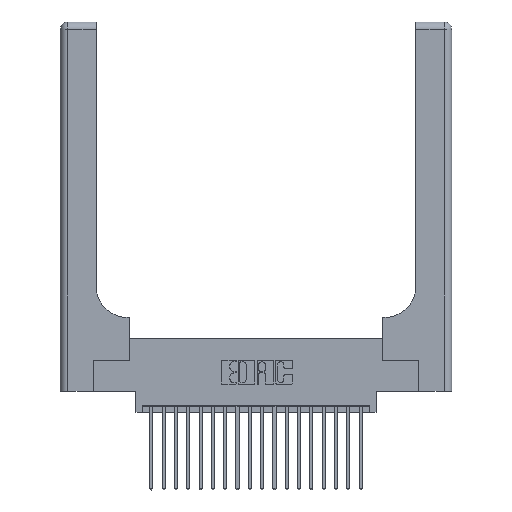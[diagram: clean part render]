
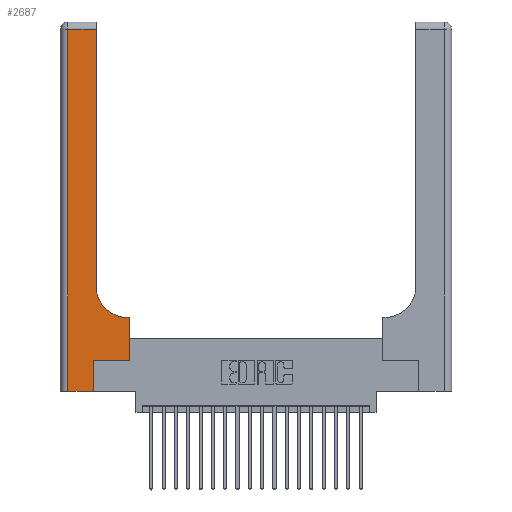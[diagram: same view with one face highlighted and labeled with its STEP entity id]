
A CAD part, top view. The second image highlights one B-rep face of the part: STEP entity #2687.
In plain terms, the highlighted planar face has unit normal (0, 0, 1).
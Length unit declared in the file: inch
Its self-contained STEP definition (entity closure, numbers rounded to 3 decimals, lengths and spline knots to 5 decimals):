
#293 = VECTOR ( 'NONE', #5653, 39.37008 ) ;
#334 = VECTOR ( 'NONE', #6214, 39.37008 ) ;
#410 = EDGE_CURVE ( 'NONE', #9413, #22531, #4582, .T. ) ;
#732 = AXIS2_PLACEMENT_3D ( 'NONE', #22303, #11913, #1393 ) ;
#791 = DIRECTION ( 'NONE',  ( 0., 0., -1. ) ) ;
#1054 = AXIS2_PLACEMENT_3D ( 'NONE', #16647, #791, #11550 ) ;
#1213 = CARTESIAN_POINT ( 'NONE',  ( 0.269, 0.25, 0.37 ) ) ;
#1229 = ORIENTED_EDGE ( 'NONE', *, *, #21513, .T. ) ;
#1301 = CARTESIAN_POINT ( 'NONE',  ( 0., 0., 0.37 ) ) ;
#1393 = DIRECTION ( 'NONE',  ( 1., 0., 0. ) ) ;
#1927 = CARTESIAN_POINT ( 'NONE',  ( 0.06, 3., 0.37 ) ) ;
#2687 = ADVANCED_FACE ( 'NONE', ( #8909 ), #16555, .F. ) ;
#2688 = CIRCLE ( 'NONE', #732, 0.25 ) ;
#2940 = VECTOR ( 'NONE', #15321, 39.37008 ) ;
#3001 = EDGE_CURVE ( 'NONE', #15989, #12633, #21549, .T. ) ;
#4472 = ORIENTED_EDGE ( 'NONE', *, *, #6084, .T. ) ;
#4482 = LINE ( 'NONE', #18387, #334 ) ;
#4582 = LINE ( 'NONE', #1301, #2940 ) ;
#4604 = CARTESIAN_POINT ( 'NONE',  ( 0.5415, 0.6, 0.37 ) ) ;
#4861 = CARTESIAN_POINT ( 'NONE',  ( 0.2915, 0.85, 0.37 ) ) ;
#5057 = VECTOR ( 'NONE', #12352, 39.37008 ) ;
#5241 = EDGE_CURVE ( 'NONE', #9313, #15313, #4482, .T. ) ;
#5549 = VERTEX_POINT ( 'NONE', #15116 ) ;
#5577 = VERTEX_POINT ( 'NONE', #4861 ) ;
#5641 = DIRECTION ( 'NONE',  ( 0., 1., 0. ) ) ;
#5653 = DIRECTION ( 'NONE',  ( -1., 0., 0. ) ) ;
#6084 = EDGE_CURVE ( 'NONE', #5549, #11121, #7155, .T. ) ;
#6214 = DIRECTION ( 'NONE',  ( -1., 0., 0. ) ) ;
#6925 = CARTESIAN_POINT ( 'NONE',  ( 0.269, 0.25, 0.37 ) ) ;
#7155 = LINE ( 'NONE', #8950, #293 ) ;
#8088 = CARTESIAN_POINT ( 'NONE',  ( 0.2915, 3., 0.37 ) ) ;
#8133 = ORIENTED_EDGE ( 'NONE', *, *, #8689, .T. ) ;
#8689 = EDGE_CURVE ( 'NONE', #5577, #5549, #21876, .T. ) ;
#8909 = FACE_OUTER_BOUND ( 'NONE', #14548, .T. ) ;
#8950 = CARTESIAN_POINT ( 'NONE',  ( 0., 2.94, 0.37 ) ) ;
#9047 = ORIENTED_EDGE ( 'NONE', *, *, #17097, .T. ) ;
#9226 = VECTOR ( 'NONE', #16979, 39.37008 ) ;
#9313 = VERTEX_POINT ( 'NONE', #21551 ) ;
#9413 = VERTEX_POINT ( 'NONE', #18988 ) ;
#11121 = VERTEX_POINT ( 'NONE', #11631 ) ;
#11384 = CARTESIAN_POINT ( 'NONE',  ( 0.269, 0., 0.37 ) ) ;
#11550 = DIRECTION ( 'NONE',  ( -1., 0., 0. ) ) ;
#11631 = CARTESIAN_POINT ( 'NONE',  ( 0.06, 2.94, 0.37 ) ) ;
#11913 = DIRECTION ( 'NONE',  ( 0., 0., -1. ) ) ;
#12352 = DIRECTION ( 'NONE',  ( 0., -1., 0. ) ) ;
#12580 = VECTOR ( 'NONE', #22347, 39.37008 ) ;
#12633 = VERTEX_POINT ( 'NONE', #12784 ) ;
#12784 = CARTESIAN_POINT ( 'NONE',  ( 0.5585, 0.25, 0.37 ) ) ;
#12981 = ORIENTED_EDGE ( 'NONE', *, *, #410, .T. ) ;
#13051 = LINE ( 'NONE', #1927, #5057 ) ;
#14033 = ORIENTED_EDGE ( 'NONE', *, *, #14092, .T. ) ;
#14092 = EDGE_CURVE ( 'NONE', #22531, #15989, #18126, .T. ) ;
#14548 = EDGE_LOOP ( 'NONE', ( #8133, #4472, #9047, #12981, #14033, #17518, #18423, #15366, #1229 ) ) ;
#15116 = CARTESIAN_POINT ( 'NONE',  ( 0.2915, 2.94, 0.37 ) ) ;
#15170 = DIRECTION ( 'NONE',  ( 0., 1., 0. ) ) ;
#15254 = CARTESIAN_POINT ( 'NONE',  ( 0.269, 0., 0.37 ) ) ;
#15313 = VERTEX_POINT ( 'NONE', #4604 ) ;
#15321 = DIRECTION ( 'NONE',  ( 1., 0., 0. ) ) ;
#15366 = ORIENTED_EDGE ( 'NONE', *, *, #5241, .T. ) ;
#15989 = VERTEX_POINT ( 'NONE', #6925 ) ;
#16425 = CARTESIAN_POINT ( 'NONE',  ( 0.5585, 0.25, 0.37 ) ) ;
#16555 = PLANE ( 'NONE',  #1054 ) ;
#16630 = LINE ( 'NONE', #16425, #17723 ) ;
#16647 = CARTESIAN_POINT ( 'NONE',  ( 0., 3., 0.37 ) ) ;
#16979 = DIRECTION ( 'NONE',  ( 1., 0., 0. ) ) ;
#17097 = EDGE_CURVE ( 'NONE', #11121, #9413, #13051, .T. ) ;
#17518 = ORIENTED_EDGE ( 'NONE', *, *, #3001, .T. ) ;
#17723 = VECTOR ( 'NONE', #5641, 39.37008 ) ;
#18126 = LINE ( 'NONE', #15254, #20029 ) ;
#18387 = CARTESIAN_POINT ( 'NONE',  ( 0.2915, 0.6, 0.37 ) ) ;
#18423 = ORIENTED_EDGE ( 'NONE', *, *, #21972, .T. ) ;
#18988 = CARTESIAN_POINT ( 'NONE',  ( 0.06, 0., 0.37 ) ) ;
#20029 = VECTOR ( 'NONE', #15170, 39.37008 ) ;
#21513 = EDGE_CURVE ( 'NONE', #15313, #5577, #2688, .T. ) ;
#21549 = LINE ( 'NONE', #1213, #9226 ) ;
#21551 = CARTESIAN_POINT ( 'NONE',  ( 0.5585, 0.6, 0.37 ) ) ;
#21876 = LINE ( 'NONE', #8088, #12580 ) ;
#21972 = EDGE_CURVE ( 'NONE', #12633, #9313, #16630, .T. ) ;
#22303 = CARTESIAN_POINT ( 'NONE',  ( 0.5415, 0.85, 0.37 ) ) ;
#22347 = DIRECTION ( 'NONE',  ( 0., 1., 0. ) ) ;
#22531 = VERTEX_POINT ( 'NONE', #11384 ) ;
